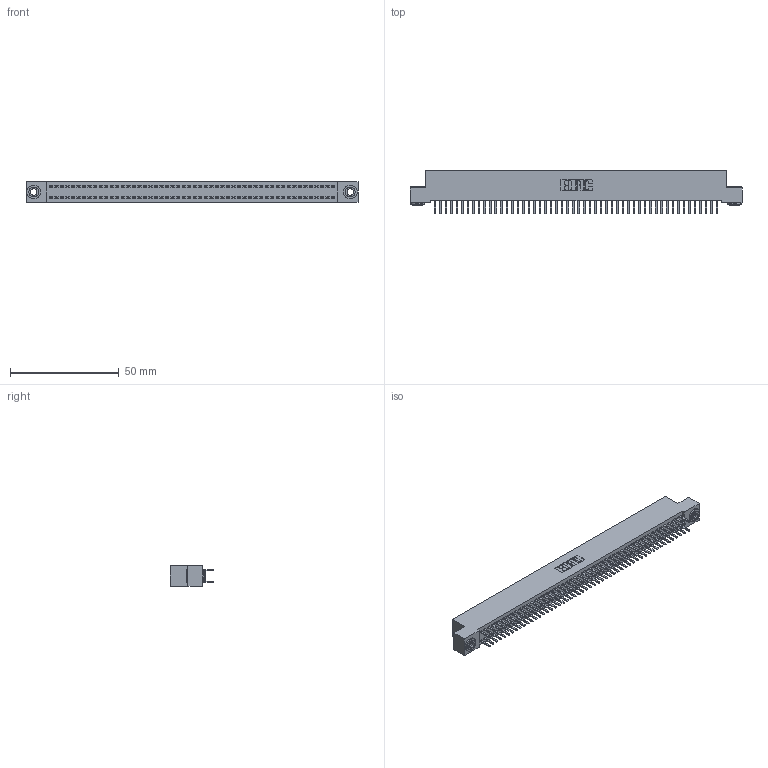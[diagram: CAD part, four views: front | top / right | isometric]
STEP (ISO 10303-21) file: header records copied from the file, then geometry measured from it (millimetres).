
FILE_DESCRIPTION (( 'STEP AP203' ), '1' );
FILE_NAME ('392-104-520-203.STEP', '2019-10-09T21:46:07', ( '' ), ( '' ), 'SwSTEP 2.0', 'SolidWorks 2016', '' );
FILE_SCHEMA (( 'CONFIG_CONTROL_DESIGN' ));
Length unit declared in the file: inch
Products named in the file (4): 392-104-520-203; 342 Part_.156 TH; 345-292-001_345-293-120; 342-250-002_345-250-002-102
Assembly tree (107 placements, depth 2):
  392-104-520-203
    342 Part_.156 TH
    345-292-001_345-293-120  x104
    342-250-002_345-250-002-102  x2
Bounding box: 152.4 x 20.02 x 9.4 mm (x, y, z)
Volume: 13717.5 mm3; surface area: 22681.4 mm2
Topology: 107 solids, 107 shells, 5972 faces, 17327 edges, 11270 vertices
Faces by surface type: plane 4028, cylinder 1936, cone 8
Entity records: 32792 total; most frequent: CARTESIAN_POINT 5409, ORIENTED_EDGE 5326, DIRECTION 4625, EDGE_CURVE 2663, VECTOR 2507, LINE 2507, VERTEX_POINT 1770, AXIS2_PLACEMENT_3D 1059
